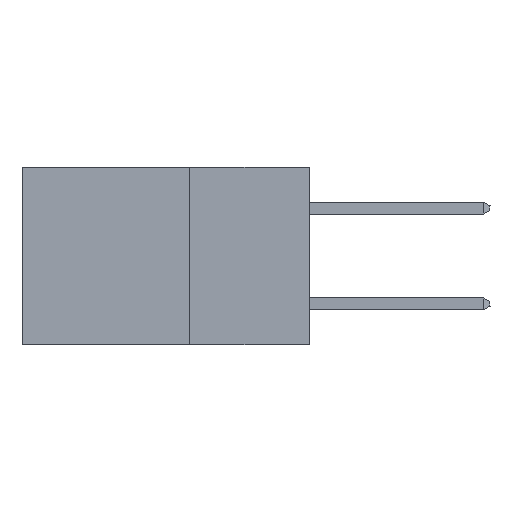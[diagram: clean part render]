
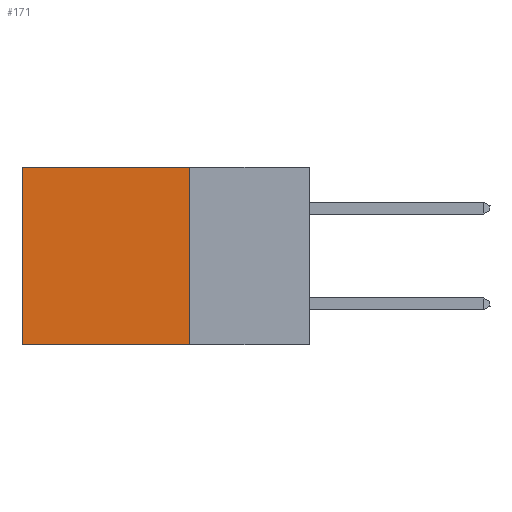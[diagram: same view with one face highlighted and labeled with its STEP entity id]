
A CAD part, left-side view. The second image highlights one B-rep face of the part: STEP entity #171.
In plain terms, the highlighted planar face has unit normal (-1, 0, 0).
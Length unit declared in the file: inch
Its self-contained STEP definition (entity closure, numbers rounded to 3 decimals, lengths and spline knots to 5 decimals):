
#171 = ADVANCED_FACE ( 'NONE', ( #2248 ), #4901, .F. ) ;
#601 = VECTOR ( 'NONE', #7689, 39.37008 ) ;
#761 = DIRECTION ( 'NONE',  ( 0., 0., -1. ) ) ;
#1071 = LINE ( 'NONE', #15874, #2185 ) ;
#1321 = VERTEX_POINT ( 'NONE', #3136 ) ;
#1426 = AXIS2_PLACEMENT_3D ( 'NONE', #15182, #16585, #761 ) ;
#1955 = VERTEX_POINT ( 'NONE', #3180 ) ;
#2066 = CARTESIAN_POINT ( 'NONE',  ( 0.2875, 0.25, 0. ) ) ;
#2185 = VECTOR ( 'NONE', #2820, 39.37008 ) ;
#2248 = FACE_OUTER_BOUND ( 'NONE', #11192, .T. ) ;
#2498 = VERTEX_POINT ( 'NONE', #6481 ) ;
#2820 = DIRECTION ( 'NONE',  ( 0., 1., 0. ) ) ;
#3136 = CARTESIAN_POINT ( 'NONE',  ( 0.2875, 0.25, -0.37 ) ) ;
#3180 = CARTESIAN_POINT ( 'NONE',  ( 0.2875, 0.6, -0.37 ) ) ;
#4185 = VECTOR ( 'NONE', #13602, 39.37008 ) ;
#4419 = ORIENTED_EDGE ( 'NONE', *, *, #10357, .T. ) ;
#4901 = PLANE ( 'NONE',  #1426 ) ;
#5177 = VECTOR ( 'NONE', #7841, 39.37008 ) ;
#5759 = EDGE_CURVE ( 'NONE', #1321, #1955, #11289, .T. ) ;
#6481 = CARTESIAN_POINT ( 'NONE',  ( 0.2875, 0.6, 0. ) ) ;
#7689 = DIRECTION ( 'NONE',  ( 0., 0., -1. ) ) ;
#7803 = LINE ( 'NONE', #17478, #4185 ) ;
#7841 = DIRECTION ( 'NONE',  ( 0., 1., 0. ) ) ;
#10215 = EDGE_CURVE ( 'NONE', #14422, #1321, #11430, .T. ) ;
#10357 = EDGE_CURVE ( 'NONE', #2498, #1955, #7803, .T. ) ;
#10996 = ORIENTED_EDGE ( 'NONE', *, *, #5759, .F. ) ;
#11192 = EDGE_LOOP ( 'NONE', ( #4419, #10996, #18581, #18673 ) ) ;
#11289 = LINE ( 'NONE', #17494, #5177 ) ;
#11430 = LINE ( 'NONE', #2066, #601 ) ;
#11574 = CARTESIAN_POINT ( 'NONE',  ( 0.2875, 0.25, 0. ) ) ;
#12717 = EDGE_CURVE ( 'NONE', #14422, #2498, #1071, .T. ) ;
#13602 = DIRECTION ( 'NONE',  ( 0., 0., -1. ) ) ;
#14422 = VERTEX_POINT ( 'NONE', #11574 ) ;
#15182 = CARTESIAN_POINT ( 'NONE',  ( 0.2875, 0.25, 0. ) ) ;
#15874 = CARTESIAN_POINT ( 'NONE',  ( 0.2875, 0.25, 0. ) ) ;
#16585 = DIRECTION ( 'NONE',  ( 1., 0., 0. ) ) ;
#17478 = CARTESIAN_POINT ( 'NONE',  ( 0.2875, 0.6, 0. ) ) ;
#17494 = CARTESIAN_POINT ( 'NONE',  ( 0.2875, 0.25, -0.37 ) ) ;
#18581 = ORIENTED_EDGE ( 'NONE', *, *, #10215, .F. ) ;
#18673 = ORIENTED_EDGE ( 'NONE', *, *, #12717, .T. ) ;
